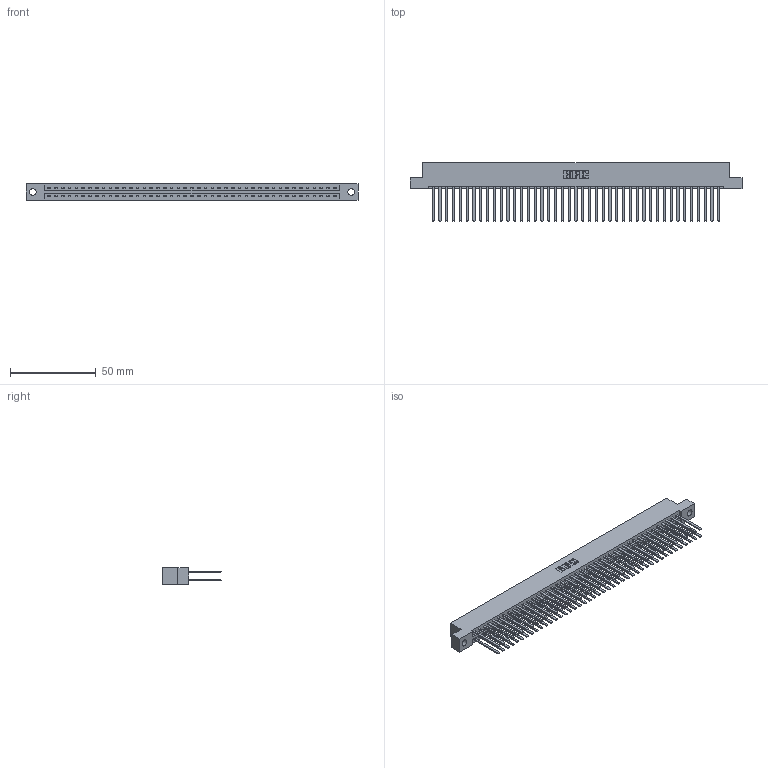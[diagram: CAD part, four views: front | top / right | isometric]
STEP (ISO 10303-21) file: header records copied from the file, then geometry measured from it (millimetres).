
FILE_DESCRIPTION (( 'STEP AP203' ), '1' );
FILE_NAME ('387-086-544-204.STEP', '2019-10-23T03:53:27', ( '' ), ( '' ), 'SwSTEP 2.0', 'SolidWorks 2016', '' );
FILE_SCHEMA (( 'CONFIG_CONTROL_DESIGN' ));
Length unit declared in the file: inch
Products named in the file (3): 345-292-001_345-293-144; 387-086-544-204; 337 Part_Flush Mounting Lugs - 0.156 Dia-TH
Assembly tree (87 placements, depth 2):
  387-086-544-204
    337 Part_Flush Mounting Lugs - 0.156 Dia-TH
    345-292-001_345-293-144  x86
Bounding box: 193.4 x 34.3 x 9.4 mm (x, y, z)
Volume: 21512.6 mm3; surface area: 28065.4 mm2
Topology: 87 solids, 87 shells, 4242 faces, 12609 edges, 8290 vertices
Faces by surface type: plane 2994, cylinder 1248
Entity records: 33029 total; most frequent: CARTESIAN_POINT 5562, ORIENTED_EDGE 5498, DIRECTION 4725, EDGE_CURVE 2749, VECTOR 2625, LINE 2625, VERTEX_POINT 1830, AXIS2_PLACEMENT_3D 1050
